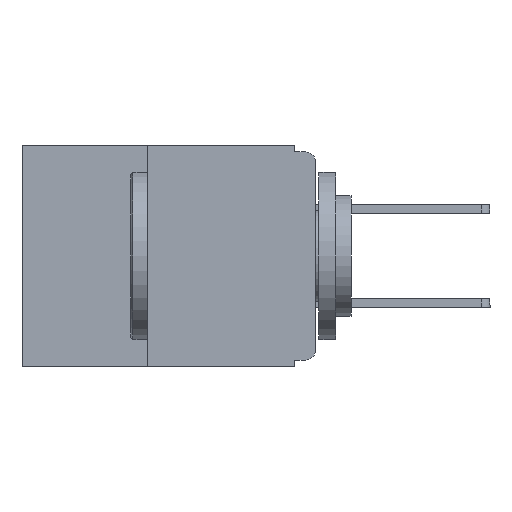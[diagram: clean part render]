
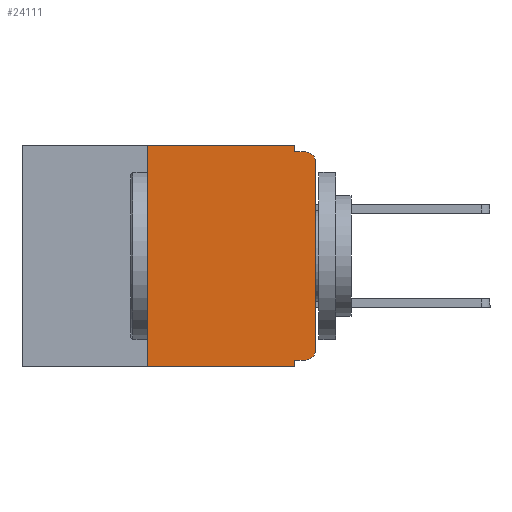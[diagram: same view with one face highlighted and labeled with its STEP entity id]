
A CAD part, left-side view. The second image highlights one B-rep face of the part: STEP entity #24111.
In plain terms, the highlighted planar face has unit normal (-1, 0, 0).
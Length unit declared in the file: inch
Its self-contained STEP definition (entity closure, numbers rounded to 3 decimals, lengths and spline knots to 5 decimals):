
#91 = CARTESIAN_POINT ( 'NONE',  ( 0., 0., -0.01 ) ) ;
#198 = VECTOR ( 'NONE', #233, 39.37008 ) ;
#233 = DIRECTION ( 'NONE',  ( 0., 0., -1. ) ) ;
#285 = LINE ( 'NONE', #91, #21171 ) ;
#690 = VERTEX_POINT ( 'NONE', #10991 ) ;
#1475 = LINE ( 'NONE', #23095, #21693 ) ;
#1583 = EDGE_CURVE ( 'NONE', #21628, #10449, #285, .T. ) ;
#2237 = ORIENTED_EDGE ( 'NONE', *, *, #1583, .F. ) ;
#2911 = DIRECTION ( 'NONE',  ( 0., 1., 0. ) ) ;
#3249 = LINE ( 'NONE', #11369, #9651 ) ;
#5262 = DIRECTION ( 'NONE',  ( 1., 0., 0. ) ) ;
#5425 = CARTESIAN_POINT ( 'NONE',  ( 0., 0.031, -0.01 ) ) ;
#5782 = ORIENTED_EDGE ( 'NONE', *, *, #24722, .T. ) ;
#5807 = CARTESIAN_POINT ( 'NONE',  ( 0., 0.015, -0.305 ) ) ;
#6035 = AXIS2_PLACEMENT_3D ( 'NONE', #12019, #11987, #11965 ) ;
#6451 = VERTEX_POINT ( 'NONE', #24161 ) ;
#7079 = CARTESIAN_POINT ( 'NONE',  ( 0., 0., -0.32 ) ) ;
#7267 = ORIENTED_EDGE ( 'NONE', *, *, #8297, .T. ) ;
#7510 = AXIS2_PLACEMENT_3D ( 'NONE', #5807, #19822, #7852 ) ;
#7852 = DIRECTION ( 'NONE',  ( 0., 0., -1. ) ) ;
#8176 = VERTEX_POINT ( 'NONE', #13185 ) ;
#8287 = DIRECTION ( 'NONE',  ( 0., 0., -1. ) ) ;
#8297 = EDGE_CURVE ( 'NONE', #6451, #10449, #18987, .T. ) ;
#8318 = ORIENTED_EDGE ( 'NONE', *, *, #12913, .F. ) ;
#8368 = EDGE_CURVE ( 'NONE', #8516, #6451, #13640, .T. ) ;
#8516 = VERTEX_POINT ( 'NONE', #9367 ) ;
#9367 = CARTESIAN_POINT ( 'NONE',  ( 0., 0., -0.305 ) ) ;
#9651 = VECTOR ( 'NONE', #10977, 39.37008 ) ;
#9768 = EDGE_CURVE ( 'NONE', #17137, #690, #21716, .T. ) ;
#10059 = ORIENTED_EDGE ( 'NONE', *, *, #8368, .T. ) ;
#10219 = CARTESIAN_POINT ( 'NONE',  ( 0., 0.437, 0. ) ) ;
#10449 = VERTEX_POINT ( 'NONE', #21314 ) ;
#10977 = DIRECTION ( 'NONE',  ( 0., 0., 1. ) ) ;
#10991 = CARTESIAN_POINT ( 'NONE',  ( 0., 0.031, -0.33 ) ) ;
#11009 = VERTEX_POINT ( 'NONE', #13890 ) ;
#11217 = EDGE_CURVE ( 'NONE', #8176, #11009, #3249, .T. ) ;
#11235 = DIRECTION ( 'NONE',  ( 0., 0., 1. ) ) ;
#11277 = CARTESIAN_POINT ( 'NONE',  ( 0., 0.437, 0. ) ) ;
#11369 = CARTESIAN_POINT ( 'NONE',  ( 0., 0.25, -0.33 ) ) ;
#11432 = CARTESIAN_POINT ( 'NONE',  ( 0., 0., 0. ) ) ;
#11792 = VECTOR ( 'NONE', #11235, 39.37008 ) ;
#11965 = DIRECTION ( 'NONE',  ( 0., 0., -1. ) ) ;
#11987 = DIRECTION ( 'NONE',  ( -1., 0., 0. ) ) ;
#12019 = CARTESIAN_POINT ( 'NONE',  ( 0., 0.015, -0.025 ) ) ;
#12117 = EDGE_CURVE ( 'NONE', #11009, #16988, #24230, .T. ) ;
#12199 = DIRECTION ( 'NONE',  ( 0., -1., 0. ) ) ;
#12433 = CARTESIAN_POINT ( 'NONE',  ( 0., 0.031, 0. ) ) ;
#12895 = VERTEX_POINT ( 'NONE', #24938 ) ;
#12913 = EDGE_CURVE ( 'NONE', #12895, #17137, #16736, .T. ) ;
#13185 = CARTESIAN_POINT ( 'NONE',  ( 0., 0.25, -0.33 ) ) ;
#13621 = VECTOR ( 'NONE', #12199, 39.37008 ) ;
#13630 = ORIENTED_EDGE ( 'NONE', *, *, #11217, .F. ) ;
#13640 = LINE ( 'NONE', #11432, #11792 ) ;
#13890 = CARTESIAN_POINT ( 'NONE',  ( 0., 0.25, 0. ) ) ;
#16157 = ORIENTED_EDGE ( 'NONE', *, *, #9768, .F. ) ;
#16487 = ORIENTED_EDGE ( 'NONE', *, *, #19539, .F. ) ;
#16736 = LINE ( 'NONE', #7079, #26005 ) ;
#16988 = VERTEX_POINT ( 'NONE', #19305 ) ;
#17137 = VERTEX_POINT ( 'NONE', #18668 ) ;
#17291 = PLANE ( 'NONE',  #21606 ) ;
#18012 = CIRCLE ( 'NONE', #7510, 0.015 ) ;
#18337 = ORIENTED_EDGE ( 'NONE', *, *, #22902, .T. ) ;
#18668 = CARTESIAN_POINT ( 'NONE',  ( 0., 0.031, -0.32 ) ) ;
#18987 = CIRCLE ( 'NONE', #6035, 0.015 ) ;
#19177 = DIRECTION ( 'NONE',  ( 0., -1., 0. ) ) ;
#19282 = DIRECTION ( 'NONE',  ( 0., 0., -1. ) ) ;
#19305 = CARTESIAN_POINT ( 'NONE',  ( 0., 0.031, 0. ) ) ;
#19539 = EDGE_CURVE ( 'NONE', #16988, #21628, #21087, .T. ) ;
#19822 = DIRECTION ( 'NONE',  ( -1., 0., 0. ) ) ;
#20544 = ORIENTED_EDGE ( 'NONE', *, *, #12117, .F. ) ;
#20782 = FACE_OUTER_BOUND ( 'NONE', #25369, .T. ) ;
#21087 = LINE ( 'NONE', #12433, #198 ) ;
#21088 = VECTOR ( 'NONE', #8287, 39.37008 ) ;
#21171 = VECTOR ( 'NONE', #24238, 39.37008 ) ;
#21314 = CARTESIAN_POINT ( 'NONE',  ( 0., 0.015, -0.01 ) ) ;
#21606 = AXIS2_PLACEMENT_3D ( 'NONE', #11277, #5262, #19282 ) ;
#21628 = VERTEX_POINT ( 'NONE', #5425 ) ;
#21693 = VECTOR ( 'NONE', #19177, 39.37008 ) ;
#21716 = LINE ( 'NONE', #22314, #21088 ) ;
#22314 = CARTESIAN_POINT ( 'NONE',  ( 0., 0.031, -0.33 ) ) ;
#22902 = EDGE_CURVE ( 'NONE', #12895, #8516, #18012, .T. ) ;
#23095 = CARTESIAN_POINT ( 'NONE',  ( 0., 0.437, -0.33 ) ) ;
#24111 = ADVANCED_FACE ( 'NONE', ( #20782 ), #17291, .F. ) ;
#24161 = CARTESIAN_POINT ( 'NONE',  ( 0., 0., -0.025 ) ) ;
#24230 = LINE ( 'NONE', #10219, #13621 ) ;
#24238 = DIRECTION ( 'NONE',  ( 0., -1., 0. ) ) ;
#24722 = EDGE_CURVE ( 'NONE', #8176, #690, #1475, .T. ) ;
#24938 = CARTESIAN_POINT ( 'NONE',  ( 0., 0.015, -0.32 ) ) ;
#25369 = EDGE_LOOP ( 'NONE', ( #10059, #7267, #2237, #16487, #20544, #13630, #5782, #16157, #8318, #18337 ) ) ;
#26005 = VECTOR ( 'NONE', #2911, 39.37008 ) ;
